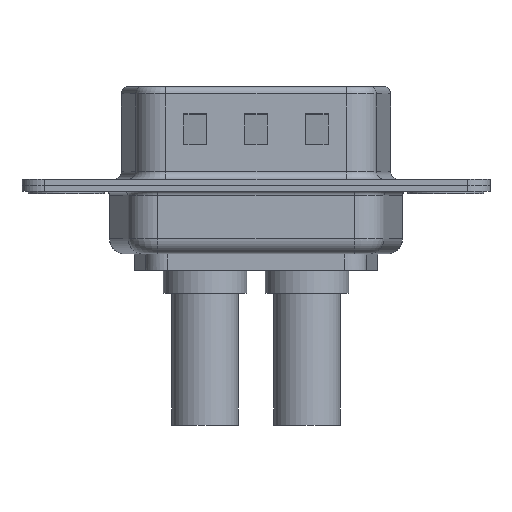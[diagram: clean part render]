
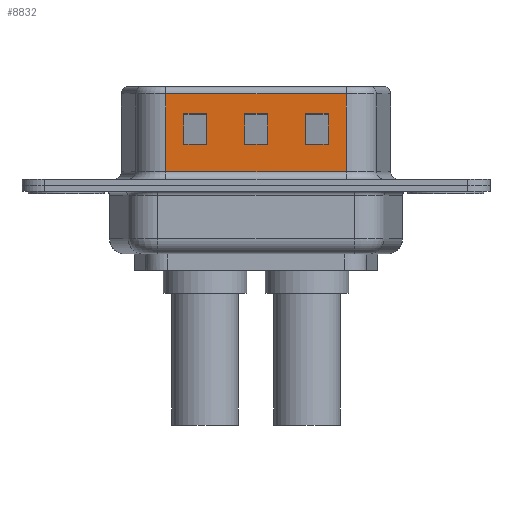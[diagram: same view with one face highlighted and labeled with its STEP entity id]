
A CAD part, front view. The second image highlights one B-rep face of the part: STEP entity #8832.
In plain terms, the highlighted planar face has unit normal (0, -1, 0).
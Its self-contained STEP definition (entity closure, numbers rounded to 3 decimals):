
#120 = CARTESIAN_POINT ( 'NONE',  ( 17.25, -4.58, 4.705 ) ) ;
#221 = LINE ( 'NONE', #7749, #12745 ) ;
#349 = ORIENTED_EDGE ( 'NONE', *, *, #1783, .T. ) ;
#525 = EDGE_LOOP ( 'NONE', ( #7839, #3478, #9562, #4510 ) ) ;
#820 = ORIENTED_EDGE ( 'NONE', *, *, #5543, .T. ) ;
#863 = FACE_BOUND ( 'NONE', #6533, .T. ) ;
#1062 = LINE ( 'NONE', #6998, #10958 ) ;
#1187 = DIRECTION ( 'NONE',  ( -1., 0., 0. ) ) ;
#1278 = DIRECTION ( 'NONE',  ( 0., 0., -1. ) ) ;
#1477 = DIRECTION ( 'NONE',  ( 0., 0., -1. ) ) ;
#1552 = CARTESIAN_POINT ( 'NONE',  ( 11.75, -4.58, 2.705 ) ) ;
#1633 = ORIENTED_EDGE ( 'NONE', *, *, #4490, .T. ) ;
#1783 = EDGE_CURVE ( 'NONE', #1955, #5879, #4607, .T. ) ;
#1834 = DIRECTION ( 'NONE',  ( 1., 0., 0. ) ) ;
#1955 = VERTEX_POINT ( 'NONE', #8151 ) ;
#2099 = VECTOR ( 'NONE', #4336, 1000. ) ;
#2432 = EDGE_LOOP ( 'NONE', ( #11237, #9607, #820, #5404 ) ) ;
#2533 = EDGE_CURVE ( 'NONE', #11086, #6028, #9401, .T. ) ;
#2537 = DIRECTION ( 'NONE',  ( 0., 0., -1. ) ) ;
#2596 = VERTEX_POINT ( 'NONE', #11065 ) ;
#3100 = VERTEX_POINT ( 'NONE', #1552 ) ;
#3104 = CARTESIAN_POINT ( 'NONE',  ( 7.75, -4.58, 6.52 ) ) ;
#3143 = EDGE_CURVE ( 'NONE', #5879, #4666, #1062, .T. ) ;
#3172 = AXIS2_PLACEMENT_3D ( 'NONE', #6084, #12764, #7083 ) ;
#3478 = ORIENTED_EDGE ( 'NONE', *, *, #10091, .T. ) ;
#3494 = EDGE_CURVE ( 'NONE', #7088, #2596, #12497, .T. ) ;
#3522 = LINE ( 'NONE', #10114, #6215 ) ;
#3572 = CARTESIAN_POINT ( 'NONE',  ( 7.75, -4.58, 2.705 ) ) ;
#3628 = ORIENTED_EDGE ( 'NONE', *, *, #5436, .T. ) ;
#3745 = LINE ( 'NONE', #8224, #8708 ) ;
#3825 = CARTESIAN_POINT ( 'NONE',  ( 14.45, -4.58, 2.705 ) ) ;
#3864 = CARTESIAN_POINT ( 'NONE',  ( 17.25, -4.58, 6.52 ) ) ;
#4038 = ORIENTED_EDGE ( 'NONE', *, *, #12481, .T. ) ;
#4074 = EDGE_CURVE ( 'NONE', #6458, #7657, #5015, .T. ) ;
#4127 = DIRECTION ( 'NONE',  ( 0., 0., 1. ) ) ;
#4186 = DIRECTION ( 'NONE',  ( 1., 0., 0. ) ) ;
#4313 = CARTESIAN_POINT ( 'NONE',  ( 18.45, -4.58, 4.705 ) ) ;
#4336 = DIRECTION ( 'NONE',  ( 0., 0., -1. ) ) ;
#4346 = EDGE_LOOP ( 'NONE', ( #3628, #7910, #10909, #5649 ) ) ;
#4490 = EDGE_CURVE ( 'NONE', #4666, #9488, #12641, .T. ) ;
#4510 = ORIENTED_EDGE ( 'NONE', *, *, #11322, .T. ) ;
#4607 = LINE ( 'NONE', #4897, #6950 ) ;
#4666 = VERTEX_POINT ( 'NONE', #8862 ) ;
#4872 = EDGE_CURVE ( 'NONE', #2596, #9535, #12191, .T. ) ;
#4897 = CARTESIAN_POINT ( 'NONE',  ( 22.45, -4.58, 2.705 ) ) ;
#5015 = LINE ( 'NONE', #8328, #12361 ) ;
#5058 = DIRECTION ( 'NONE',  ( 1., 0., 0. ) ) ;
#5192 = VERTEX_POINT ( 'NONE', #9492 ) ;
#5404 = ORIENTED_EDGE ( 'NONE', *, *, #6859, .T. ) ;
#5436 = EDGE_CURVE ( 'NONE', #5484, #5192, #12179, .T. ) ;
#5484 = VERTEX_POINT ( 'NONE', #8481 ) ;
#5494 = CARTESIAN_POINT ( 'NONE',  ( 18.45, -4.58, 6.02 ) ) ;
#5543 = EDGE_CURVE ( 'NONE', #9535, #3100, #3522, .T. ) ;
#5613 = VECTOR ( 'NONE', #4186, 1000. ) ;
#5649 = ORIENTED_EDGE ( 'NONE', *, *, #10628, .T. ) ;
#5711 = CARTESIAN_POINT ( 'NONE',  ( 14.45, -4.58, 4.705 ) ) ;
#5879 = VERTEX_POINT ( 'NONE', #12102 ) ;
#5948 = LINE ( 'NONE', #3864, #8272 ) ;
#6022 = CARTESIAN_POINT ( 'NONE',  ( 22.45, -4.58, 4.705 ) ) ;
#6028 = VERTEX_POINT ( 'NONE', #7144 ) ;
#6084 = CARTESIAN_POINT ( 'NONE',  ( 18.45, -4.58, 6.52 ) ) ;
#6160 = VECTOR ( 'NONE', #9727, 1000. ) ;
#6215 = VECTOR ( 'NONE', #10326, 1000. ) ;
#6295 = FACE_BOUND ( 'NONE', #4346, .T. ) ;
#6458 = VERTEX_POINT ( 'NONE', #8623 ) ;
#6533 = EDGE_LOOP ( 'NONE', ( #4038, #349, #10240, #1633 ) ) ;
#6609 = CARTESIAN_POINT ( 'NONE',  ( 18.45, -4.58, 6.52 ) ) ;
#6859 = EDGE_CURVE ( 'NONE', #3100, #7088, #221, .T. ) ;
#6901 = VERTEX_POINT ( 'NONE', #3572 ) ;
#6950 = VECTOR ( 'NONE', #12649, 1000. ) ;
#6983 = DIRECTION ( 'NONE',  ( 0., 0., 1. ) ) ;
#6998 = CARTESIAN_POINT ( 'NONE',  ( 15.75, -4.58, 6.52 ) ) ;
#7083 = DIRECTION ( 'NONE',  ( 0., 0., 1. ) ) ;
#7088 = VERTEX_POINT ( 'NONE', #10842 ) ;
#7144 = CARTESIAN_POINT ( 'NONE',  ( 18.45, -4.58, 0.9 ) ) ;
#7351 = VECTOR ( 'NONE', #4127, 1000. ) ;
#7432 = CARTESIAN_POINT ( 'NONE',  ( 9.25, -4.58, 6.52 ) ) ;
#7657 = VERTEX_POINT ( 'NONE', #9822 ) ;
#7704 = VECTOR ( 'NONE', #9608, 1000. ) ;
#7749 = CARTESIAN_POINT ( 'NONE',  ( 11.75, -4.58, 6.52 ) ) ;
#7839 = ORIENTED_EDGE ( 'NONE', *, *, #2533, .F. ) ;
#7841 = VECTOR ( 'NONE', #5058, 1000. ) ;
#7910 = ORIENTED_EDGE ( 'NONE', *, *, #8086, .T. ) ;
#8086 = EDGE_CURVE ( 'NONE', #5192, #6901, #8757, .T. ) ;
#8151 = CARTESIAN_POINT ( 'NONE',  ( 17.25, -4.58, 2.705 ) ) ;
#8224 = CARTESIAN_POINT ( 'NONE',  ( 18.45, -4.58, 6.02 ) ) ;
#8272 = VECTOR ( 'NONE', #12520, 1000. ) ;
#8328 = CARTESIAN_POINT ( 'NONE',  ( 6.55, -4.58, 6.52 ) ) ;
#8479 = CARTESIAN_POINT ( 'NONE',  ( 7.75, -4.58, 4.705 ) ) ;
#8481 = CARTESIAN_POINT ( 'NONE',  ( 9.25, -4.58, 4.705 ) ) ;
#8623 = CARTESIAN_POINT ( 'NONE',  ( 6.55, -4.58, 6.02 ) ) ;
#8708 = VECTOR ( 'NONE', #1187, 1000. ) ;
#8757 = LINE ( 'NONE', #3825, #6160 ) ;
#8832 = ADVANCED_FACE ( 'NONE', ( #6295, #863, #11673, #11099 ), #9956, .F. ) ;
#8862 = CARTESIAN_POINT ( 'NONE',  ( 15.75, -4.58, 4.705 ) ) ;
#9296 = CARTESIAN_POINT ( 'NONE',  ( 13.25, -4.58, 2.705 ) ) ;
#9401 = LINE ( 'NONE', #6609, #11542 ) ;
#9488 = VERTEX_POINT ( 'NONE', #120 ) ;
#9492 = CARTESIAN_POINT ( 'NONE',  ( 9.25, -4.58, 2.705 ) ) ;
#9535 = VERTEX_POINT ( 'NONE', #9296 ) ;
#9562 = ORIENTED_EDGE ( 'NONE', *, *, #4074, .T. ) ;
#9607 = ORIENTED_EDGE ( 'NONE', *, *, #4872, .T. ) ;
#9608 = DIRECTION ( 'NONE',  ( 1., 0., 0. ) ) ;
#9727 = DIRECTION ( 'NONE',  ( -1., 0., 0. ) ) ;
#9729 = VECTOR ( 'NONE', #1278, 1000. ) ;
#9822 = CARTESIAN_POINT ( 'NONE',  ( 6.55, -4.58, 0.9 ) ) ;
#9956 = PLANE ( 'NONE',  #3172 ) ;
#9988 = EDGE_CURVE ( 'NONE', #6901, #11685, #12674, .T. ) ;
#10036 = VECTOR ( 'NONE', #1834, 1000. ) ;
#10091 = EDGE_CURVE ( 'NONE', #11086, #6458, #3745, .T. ) ;
#10114 = CARTESIAN_POINT ( 'NONE',  ( 18.45, -4.58, 2.705 ) ) ;
#10240 = ORIENTED_EDGE ( 'NONE', *, *, #3143, .T. ) ;
#10326 = DIRECTION ( 'NONE',  ( -1., 0., 0. ) ) ;
#10366 = LINE ( 'NONE', #10845, #7841 ) ;
#10538 = LINE ( 'NONE', #5711, #7704 ) ;
#10628 = EDGE_CURVE ( 'NONE', #11685, #5484, #10538, .T. ) ;
#10842 = CARTESIAN_POINT ( 'NONE',  ( 11.75, -4.58, 4.705 ) ) ;
#10845 = CARTESIAN_POINT ( 'NONE',  ( 18.45, -4.58, 0.9 ) ) ;
#10909 = ORIENTED_EDGE ( 'NONE', *, *, #9988, .T. ) ;
#10958 = VECTOR ( 'NONE', #6983, 1000. ) ;
#11065 = CARTESIAN_POINT ( 'NONE',  ( 13.25, -4.58, 4.705 ) ) ;
#11086 = VERTEX_POINT ( 'NONE', #5494 ) ;
#11099 = FACE_OUTER_BOUND ( 'NONE', #525, .T. ) ;
#11237 = ORIENTED_EDGE ( 'NONE', *, *, #3494, .T. ) ;
#11322 = EDGE_CURVE ( 'NONE', #7657, #6028, #10366, .T. ) ;
#11403 = CARTESIAN_POINT ( 'NONE',  ( 13.25, -4.58, 6.52 ) ) ;
#11542 = VECTOR ( 'NONE', #2537, 1000. ) ;
#11673 = FACE_BOUND ( 'NONE', #2432, .T. ) ;
#11685 = VERTEX_POINT ( 'NONE', #8479 ) ;
#12102 = CARTESIAN_POINT ( 'NONE',  ( 15.75, -4.58, 2.705 ) ) ;
#12179 = LINE ( 'NONE', #7432, #2099 ) ;
#12191 = LINE ( 'NONE', #11403, #9729 ) ;
#12356 = DIRECTION ( 'NONE',  ( 0., 0., 1. ) ) ;
#12361 = VECTOR ( 'NONE', #1477, 1000. ) ;
#12481 = EDGE_CURVE ( 'NONE', #9488, #1955, #5948, .T. ) ;
#12497 = LINE ( 'NONE', #4313, #10036 ) ;
#12520 = DIRECTION ( 'NONE',  ( 0., 0., -1. ) ) ;
#12641 = LINE ( 'NONE', #6022, #5613 ) ;
#12649 = DIRECTION ( 'NONE',  ( -1., 0., 0. ) ) ;
#12674 = LINE ( 'NONE', #3104, #7351 ) ;
#12745 = VECTOR ( 'NONE', #12356, 1000. ) ;
#12764 = DIRECTION ( 'NONE',  ( 0., 1., 0. ) ) ;
